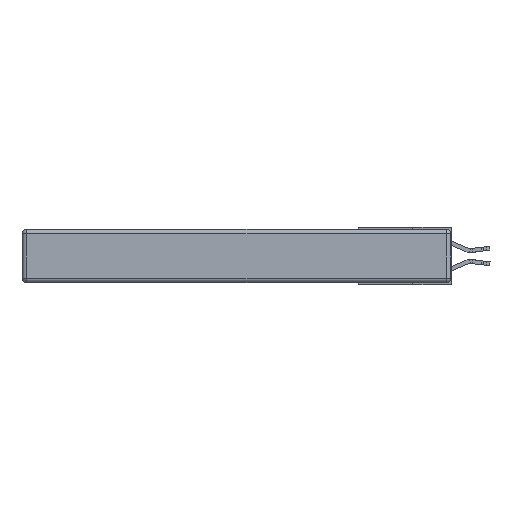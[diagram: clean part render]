
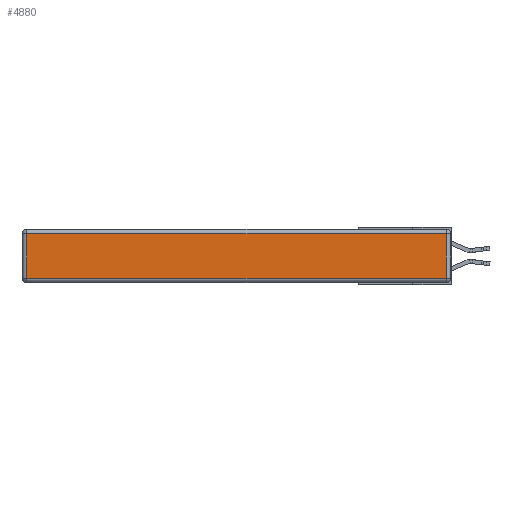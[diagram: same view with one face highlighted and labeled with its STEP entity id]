
A CAD part, left-side view. The second image highlights one B-rep face of the part: STEP entity #4880.
In plain terms, the highlighted planar face has unit normal (-1, 0, 0).
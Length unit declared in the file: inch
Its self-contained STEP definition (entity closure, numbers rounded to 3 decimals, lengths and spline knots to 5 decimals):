
#762 = PLANE ( 'NONE',  #24198 ) ;
#1955 = VERTEX_POINT ( 'NONE', #15414 ) ;
#2678 = EDGE_CURVE ( 'NONE', #30806, #1955, #27876, .T. ) ;
#3515 = VERTEX_POINT ( 'NONE', #5093 ) ;
#4576 = CARTESIAN_POINT ( 'NONE',  ( 0., 0.03, -0.343 ) ) ;
#4880 = ADVANCED_FACE ( 'NONE', ( #16580 ), #762, .T. ) ;
#5093 = CARTESIAN_POINT ( 'NONE',  ( 0., 2.72, -0.03 ) ) ;
#5808 = DIRECTION ( 'NONE',  ( 0., 0., -1. ) ) ;
#7065 = VECTOR ( 'NONE', #22153, 39.37008 ) ;
#8132 = ORIENTED_EDGE ( 'NONE', *, *, #2678, .T. ) ;
#8929 = ORIENTED_EDGE ( 'NONE', *, *, #13445, .T. ) ;
#10889 = LINE ( 'NONE', #31630, #28827 ) ;
#12721 = LINE ( 'NONE', #17149, #7065 ) ;
#13445 = EDGE_CURVE ( 'NONE', #1955, #20974, #22099, .T. ) ;
#13974 = ORIENTED_EDGE ( 'NONE', *, *, #21360, .T. ) ;
#15414 = CARTESIAN_POINT ( 'NONE',  ( 0., 0.03, -0.313 ) ) ;
#16196 = DIRECTION ( 'NONE',  ( -1., 0., 0. ) ) ;
#16580 = FACE_OUTER_BOUND ( 'NONE', #30772, .T. ) ;
#17149 = CARTESIAN_POINT ( 'NONE',  ( 0., 2.75, -0.03 ) ) ;
#18311 = VECTOR ( 'NONE', #30669, 39.37008 ) ;
#18766 = EDGE_CURVE ( 'NONE', #3515, #30806, #10889, .T. ) ;
#18849 = CARTESIAN_POINT ( 'NONE',  ( 0., 0., -0.343 ) ) ;
#19773 = ORIENTED_EDGE ( 'NONE', *, *, #18766, .T. ) ;
#20175 = CARTESIAN_POINT ( 'NONE',  ( 0., 0., -0.313 ) ) ;
#20974 = VERTEX_POINT ( 'NONE', #24113 ) ;
#21360 = EDGE_CURVE ( 'NONE', #20974, #3515, #12721, .T. ) ;
#22099 = LINE ( 'NONE', #4576, #24866 ) ;
#22153 = DIRECTION ( 'NONE',  ( 0., 1., 0. ) ) ;
#22444 = DIRECTION ( 'NONE',  ( 0., 0., 1. ) ) ;
#24113 = CARTESIAN_POINT ( 'NONE',  ( 0., 0.03, -0.03 ) ) ;
#24198 = AXIS2_PLACEMENT_3D ( 'NONE', #18849, #16196, #29110 ) ;
#24866 = VECTOR ( 'NONE', #22444, 39.37008 ) ;
#27876 = LINE ( 'NONE', #20175, #18311 ) ;
#28827 = VECTOR ( 'NONE', #5808, 39.37008 ) ;
#29110 = DIRECTION ( 'NONE',  ( 0., 0., 1. ) ) ;
#29700 = CARTESIAN_POINT ( 'NONE',  ( 0., 2.72, -0.313 ) ) ;
#30669 = DIRECTION ( 'NONE',  ( 0., -1., 0. ) ) ;
#30772 = EDGE_LOOP ( 'NONE', ( #8132, #8929, #13974, #19773 ) ) ;
#30806 = VERTEX_POINT ( 'NONE', #29700 ) ;
#31630 = CARTESIAN_POINT ( 'NONE',  ( 0., 2.72, -0.343 ) ) ;
